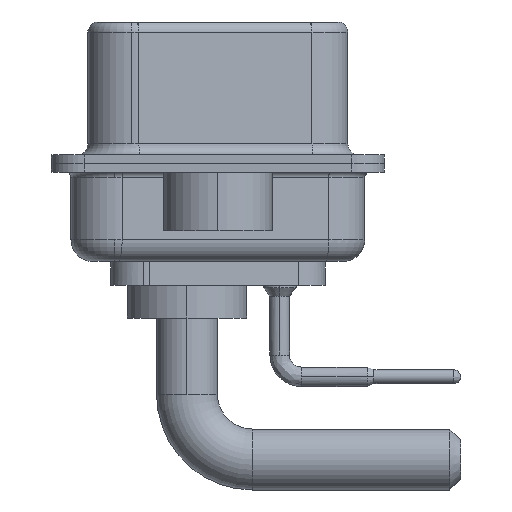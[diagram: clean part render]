
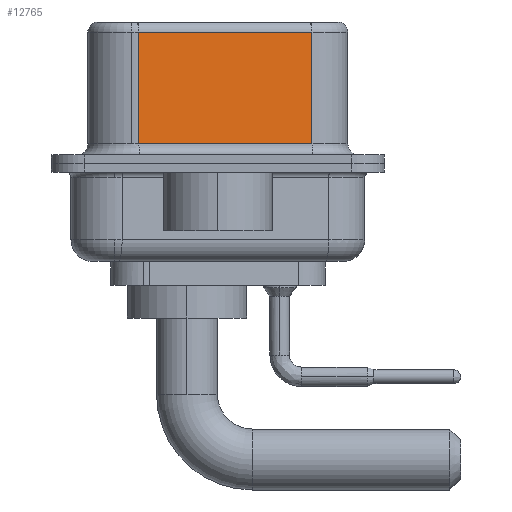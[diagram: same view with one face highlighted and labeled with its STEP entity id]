
A CAD part, left-side view. The second image highlights one B-rep face of the part: STEP entity #12765.
In plain terms, the highlighted planar face has unit normal (-0.985, -0.174, 0).
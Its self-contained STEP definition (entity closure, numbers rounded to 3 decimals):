
#1052 = CARTESIAN_POINT ( 'NONE',  ( 3.73, 3.628, 6.52 ) ) ;
#2214 = EDGE_CURVE ( 'NONE', #6856, #11604, #21811, .T. ) ;
#3129 = PLANE ( 'NONE',  #7346 ) ;
#3254 = CARTESIAN_POINT ( 'NONE',  ( 5.132, -4.322, 6.52 ) ) ;
#3472 = DIRECTION ( 'NONE',  ( -0.174, 0.985, 0. ) ) ;
#3935 = VECTOR ( 'NONE', #19800, 1000. ) ;
#4860 = CARTESIAN_POINT ( 'NONE',  ( 5.132, -4.322, 0.9 ) ) ;
#5225 = CARTESIAN_POINT ( 'NONE',  ( 5.132, -4.322, 6.52 ) ) ;
#5278 = EDGE_CURVE ( 'NONE', #23759, #11604, #21455, .T. ) ;
#5340 = DIRECTION ( 'NONE',  ( 0., 0., -1. ) ) ;
#6131 = VECTOR ( 'NONE', #8849, 1000. ) ;
#6856 = VERTEX_POINT ( 'NONE', #11952 ) ;
#7346 = AXIS2_PLACEMENT_3D ( 'NONE', #3254, #16432, #10627 ) ;
#8811 = LINE ( 'NONE', #20049, #13017 ) ;
#8849 = DIRECTION ( 'NONE',  ( 0.174, -0.985, 0. ) ) ;
#10627 = DIRECTION ( 'NONE',  ( -0.174, 0.985, 0. ) ) ;
#10862 = EDGE_CURVE ( 'NONE', #13543, #23759, #21387, .T. ) ;
#11012 = CARTESIAN_POINT ( 'NONE',  ( 3.73, 3.628, 6.02 ) ) ;
#11604 = VERTEX_POINT ( 'NONE', #16984 ) ;
#11952 = CARTESIAN_POINT ( 'NONE',  ( 5.132, -4.322, 6.02 ) ) ;
#12765 = ADVANCED_FACE ( 'NONE', ( #16076 ), #3129, .F. ) ;
#13017 = VECTOR ( 'NONE', #3472, 1000. ) ;
#13543 = VERTEX_POINT ( 'NONE', #11012 ) ;
#14716 = EDGE_CURVE ( 'NONE', #6856, #13543, #8811, .T. ) ;
#15150 = ORIENTED_EDGE ( 'NONE', *, *, #2214, .F. ) ;
#15391 = ORIENTED_EDGE ( 'NONE', *, *, #5278, .T. ) ;
#16076 = FACE_OUTER_BOUND ( 'NONE', #19334, .T. ) ;
#16432 = DIRECTION ( 'NONE',  ( 0.985, 0.174, 0. ) ) ;
#16777 = VECTOR ( 'NONE', #5340, 1000. ) ;
#16984 = CARTESIAN_POINT ( 'NONE',  ( 5.132, -4.322, 0.9 ) ) ;
#17428 = CARTESIAN_POINT ( 'NONE',  ( 3.73, 3.628, 0.9 ) ) ;
#17733 = ORIENTED_EDGE ( 'NONE', *, *, #14716, .T. ) ;
#19334 = EDGE_LOOP ( 'NONE', ( #15150, #17733, #21218, #15391 ) ) ;
#19800 = DIRECTION ( 'NONE',  ( 0., 0., -1. ) ) ;
#20049 = CARTESIAN_POINT ( 'NONE',  ( 5.132, -4.322, 6.02 ) ) ;
#21218 = ORIENTED_EDGE ( 'NONE', *, *, #10862, .T. ) ;
#21387 = LINE ( 'NONE', #1052, #3935 ) ;
#21455 = LINE ( 'NONE', #4860, #6131 ) ;
#21811 = LINE ( 'NONE', #5225, #16777 ) ;
#23759 = VERTEX_POINT ( 'NONE', #17428 ) ;
